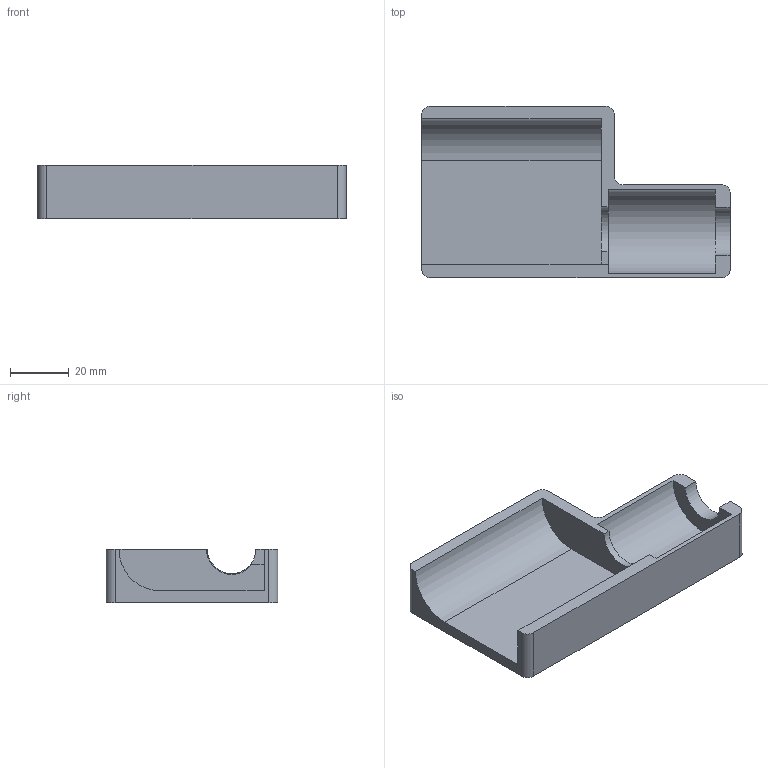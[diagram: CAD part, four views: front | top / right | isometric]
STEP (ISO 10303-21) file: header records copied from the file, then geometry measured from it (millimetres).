
FILE_DESCRIPTION(/* description */ (''),/* implementation_level */ '2;1');
FILE_NAME(/* name */ 'FGC-9_MkII_Headspacing_Jig.step',/* time_stamp */ '2021-03-26T15:13:35+01:00',/* author */ (''),/* organization */ (''),/* preprocessor_version */ 'ST-DEVELOPER v18.1',/* originating_system */ 'Autodesk Translation Framework v9.10.0.1330',/* authorisation */ '');
FILE_SCHEMA (('AUTOMOTIVE_DESIGN { 1 0 10303 214 3 1 1 }'));
Length unit declared in the file: millimetre
Products named in the file (2): FGC-9_MkII_Headspacing_Jig; FGC-9_MkII_Headspacing_Jig_1
Assembly tree (1 placements, depth 2):
  FGC-9_MkII_Headspacing_Jig
    FGC-9_MkII_Headspacing_Jig_1
Bounding box: 104.76 x 58.29 x 18.1 mm (x, y, z)
Volume: 39309.7 mm3; surface area: 18024.9 mm2
Topology: 1 solids, 1 shells, 25 faces, 69 edges, 46 vertices
Faces by surface type: plane 15, cylinder 10
Entity records: 863 total; most frequent: DIRECTION 145, CARTESIAN_POINT 143, ORIENTED_EDGE 138, EDGE_CURVE 69, LINE 49, VECTOR 49, AXIS2_PLACEMENT_3D 48, VERTEX_POINT 46
